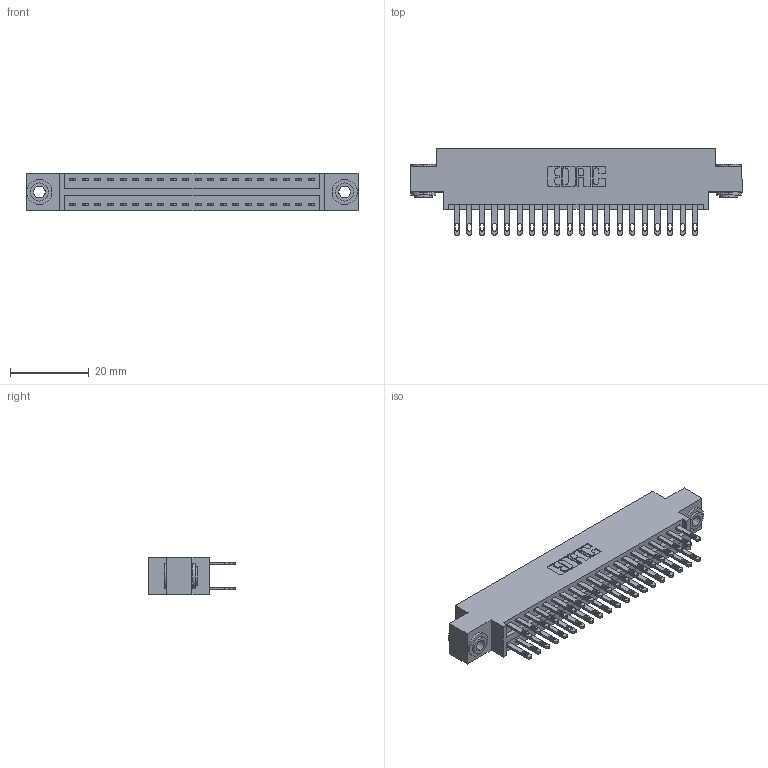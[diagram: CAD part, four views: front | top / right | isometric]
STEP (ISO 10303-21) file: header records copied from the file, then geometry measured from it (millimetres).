
FILE_DESCRIPTION (( 'STEP AP203' ), '1' );
FILE_NAME ('896-040-500-803.STEP', '2021-07-27T21:14:43', ( '' ), ( '' ), 'SwSTEP 2.0', 'SolidWorks 2020', '' );
FILE_SCHEMA (( 'CONFIG_CONTROL_DESIGN' ));
Length unit declared in the file: inch
Products named in the file (4): 345-250-002_345-250-002-102; 846 Part_0.170 Offset - 0.156 Dia-TH; 896-040-500-803; 345-292-001_345-293-100
Assembly tree (43 placements, depth 2):
  896-040-500-803
    846 Part_0.170 Offset - 0.156 Dia-TH
    345-292-001_345-293-100  x40
    345-250-002_345-250-002-102  x2
Bounding box: 84.07 x 21.84 x 9.4 mm (x, y, z)
Volume: 8014.4 mm3; surface area: 11483 mm2
Topology: 43 solids, 43 shells, 2084 faces, 6297 edges, 4194 vertices
Faces by surface type: plane 1250, cylinder 826, cone 8
Entity records: 16726 total; most frequent: CARTESIAN_POINT 2763, ORIENTED_EDGE 2690, DIRECTION 2519, EDGE_CURVE 1345, LINE 1105, VECTOR 1105, VERTEX_POINT 894, AXIS2_PLACEMENT_3D 707
